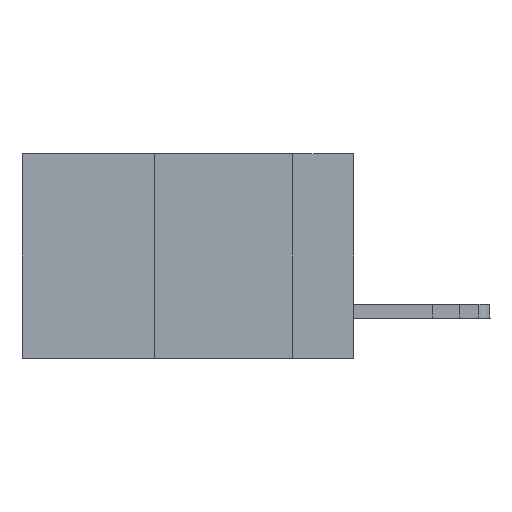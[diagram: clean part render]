
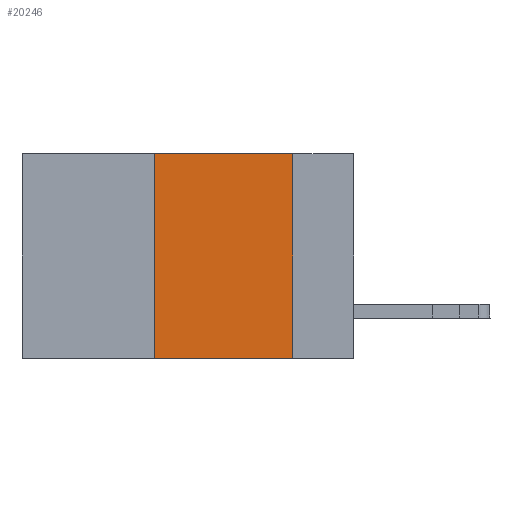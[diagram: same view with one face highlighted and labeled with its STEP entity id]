
A CAD part, left-side view. The second image highlights one B-rep face of the part: STEP entity #20246.
In plain terms, the highlighted planar face has unit normal (-1, 0, 0).
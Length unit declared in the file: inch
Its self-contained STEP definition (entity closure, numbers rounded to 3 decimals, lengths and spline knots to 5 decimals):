
#220 = LINE ( 'NONE', #2977, #747 ) ;
#294 = CARTESIAN_POINT ( 'NONE',  ( 0., 0.6, -0.37 ) ) ;
#673 = LINE ( 'NONE', #7959, #6776 ) ;
#740 = CARTESIAN_POINT ( 'NONE',  ( 0., 0.11, 0. ) ) ;
#747 = VECTOR ( 'NONE', #7789, 39.37008 ) ;
#1328 = DIRECTION ( 'NONE',  ( 0., -1., 0. ) ) ;
#1727 = EDGE_CURVE ( 'NONE', #16194, #15574, #220, .T. ) ;
#1808 = CARTESIAN_POINT ( 'NONE',  ( 0., 0.36, 0. ) ) ;
#2370 = VECTOR ( 'NONE', #13226, 39.37008 ) ;
#2977 = CARTESIAN_POINT ( 'NONE',  ( 0., 0.11, 0. ) ) ;
#4106 = LINE ( 'NONE', #294, #18413 ) ;
#4932 = EDGE_LOOP ( 'NONE', ( #6612, #18983, #13396, #19540 ) ) ;
#5869 = DIRECTION ( 'NONE',  ( 0., -1., 0. ) ) ;
#6612 = ORIENTED_EDGE ( 'NONE', *, *, #1727, .F. ) ;
#6776 = VECTOR ( 'NONE', #5869, 39.37008 ) ;
#6793 = DIRECTION ( 'NONE',  ( 1., 0., 0. ) ) ;
#6864 = DIRECTION ( 'NONE',  ( 0., 0., -1. ) ) ;
#6935 = PLANE ( 'NONE',  #11128 ) ;
#7175 = CARTESIAN_POINT ( 'NONE',  ( 0., 0.36, 0. ) ) ;
#7789 = DIRECTION ( 'NONE',  ( 0., 0., -1. ) ) ;
#7959 = CARTESIAN_POINT ( 'NONE',  ( 0., 0.6, 0. ) ) ;
#8827 = CARTESIAN_POINT ( 'NONE',  ( 0., 0.11, -0.37 ) ) ;
#11128 = AXIS2_PLACEMENT_3D ( 'NONE', #16520, #6793, #6864 ) ;
#11458 = CARTESIAN_POINT ( 'NONE',  ( 0., 0.36, -0.37 ) ) ;
#12423 = VERTEX_POINT ( 'NONE', #7175 ) ;
#12599 = VERTEX_POINT ( 'NONE', #11458 ) ;
#13150 = EDGE_CURVE ( 'NONE', #12599, #15574, #4106, .T. ) ;
#13226 = DIRECTION ( 'NONE',  ( 0., 0., 1. ) ) ;
#13396 = ORIENTED_EDGE ( 'NONE', *, *, #20080, .F. ) ;
#15574 = VERTEX_POINT ( 'NONE', #8827 ) ;
#16194 = VERTEX_POINT ( 'NONE', #740 ) ;
#16421 = FACE_OUTER_BOUND ( 'NONE', #4932, .T. ) ;
#16520 = CARTESIAN_POINT ( 'NONE',  ( 0., 0.6, 0. ) ) ;
#18413 = VECTOR ( 'NONE', #1328, 39.37008 ) ;
#18565 = EDGE_CURVE ( 'NONE', #12423, #16194, #673, .T. ) ;
#18937 = LINE ( 'NONE', #1808, #2370 ) ;
#18983 = ORIENTED_EDGE ( 'NONE', *, *, #18565, .F. ) ;
#19540 = ORIENTED_EDGE ( 'NONE', *, *, #13150, .T. ) ;
#20080 = EDGE_CURVE ( 'NONE', #12599, #12423, #18937, .T. ) ;
#20246 = ADVANCED_FACE ( 'NONE', ( #16421 ), #6935, .F. ) ;
